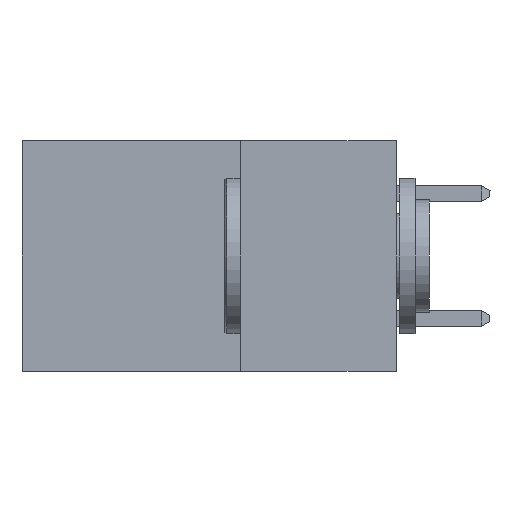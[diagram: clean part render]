
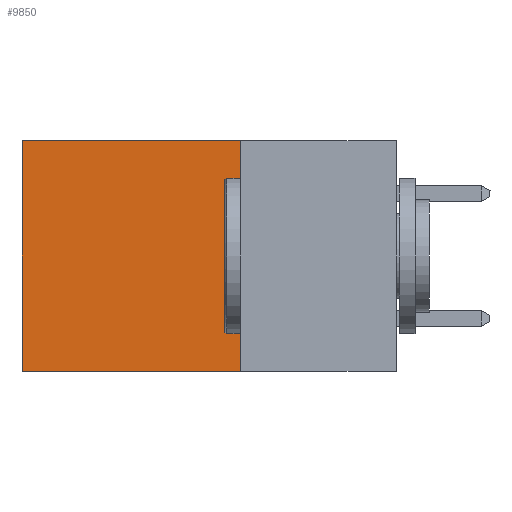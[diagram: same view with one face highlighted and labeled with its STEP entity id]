
A CAD part, left-side view. The second image highlights one B-rep face of the part: STEP entity #9850.
In plain terms, the highlighted planar face has unit normal (-1, 0, 0).
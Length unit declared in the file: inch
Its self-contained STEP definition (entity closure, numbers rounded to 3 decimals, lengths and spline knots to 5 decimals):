
#360 = EDGE_LOOP ( 'NONE', ( #5847, #7044, #11346, #6900 ) ) ;
#892 = DIRECTION ( 'NONE',  ( 1., 0., 0. ) ) ;
#955 = LINE ( 'NONE', #7389, #6560 ) ;
#984 = VERTEX_POINT ( 'NONE', #8014 ) ;
#1682 = AXIS2_PLACEMENT_3D ( 'NONE', #8633, #892, #7744 ) ;
#2180 = CARTESIAN_POINT ( 'NONE',  ( 0.298, 0.25, 0. ) ) ;
#2944 = EDGE_CURVE ( 'NONE', #7789, #984, #8192, .T. ) ;
#3063 = CARTESIAN_POINT ( 'NONE',  ( 0.298, 0.25, 0. ) ) ;
#3482 = LINE ( 'NONE', #5818, #8263 ) ;
#4239 = LINE ( 'NONE', #2180, #6195 ) ;
#5123 = VERTEX_POINT ( 'NONE', #5521 ) ;
#5280 = EDGE_CURVE ( 'NONE', #8466, #7789, #955, .T. ) ;
#5521 = CARTESIAN_POINT ( 'NONE',  ( 0.298, 0.25, -0.37 ) ) ;
#5671 = DIRECTION ( 'NONE',  ( 0., 0., -1. ) ) ;
#5818 = CARTESIAN_POINT ( 'NONE',  ( 0.298, 0.25, -0.37 ) ) ;
#5847 = ORIENTED_EDGE ( 'NONE', *, *, #2944, .T. ) ;
#6195 = VECTOR ( 'NONE', #7963, 39.37008 ) ;
#6253 = CARTESIAN_POINT ( 'NONE',  ( 0.298, 0.6, 0. ) ) ;
#6560 = VECTOR ( 'NONE', #9180, 39.37008 ) ;
#6900 = ORIENTED_EDGE ( 'NONE', *, *, #5280, .T. ) ;
#6981 = FACE_OUTER_BOUND ( 'NONE', #360, .T. ) ;
#7044 = ORIENTED_EDGE ( 'NONE', *, *, #10268, .F. ) ;
#7389 = CARTESIAN_POINT ( 'NONE',  ( 0.298, 0.25, 0. ) ) ;
#7744 = DIRECTION ( 'NONE',  ( 0., 0., -1. ) ) ;
#7789 = VERTEX_POINT ( 'NONE', #9794 ) ;
#7963 = DIRECTION ( 'NONE',  ( 0., 0., -1. ) ) ;
#8014 = CARTESIAN_POINT ( 'NONE',  ( 0.298, 0.6, -0.37 ) ) ;
#8192 = LINE ( 'NONE', #6253, #9104 ) ;
#8263 = VECTOR ( 'NONE', #10563, 39.37008 ) ;
#8466 = VERTEX_POINT ( 'NONE', #3063 ) ;
#8633 = CARTESIAN_POINT ( 'NONE',  ( 0.298, 0.25, 0. ) ) ;
#9104 = VECTOR ( 'NONE', #5671, 39.37008 ) ;
#9180 = DIRECTION ( 'NONE',  ( 0., 1., 0. ) ) ;
#9794 = CARTESIAN_POINT ( 'NONE',  ( 0.298, 0.6, 0. ) ) ;
#9850 = ADVANCED_FACE ( 'NONE', ( #6981 ), #12462, .F. ) ;
#10268 = EDGE_CURVE ( 'NONE', #5123, #984, #3482, .T. ) ;
#10563 = DIRECTION ( 'NONE',  ( 0., 1., 0. ) ) ;
#11346 = ORIENTED_EDGE ( 'NONE', *, *, #11757, .F. ) ;
#11757 = EDGE_CURVE ( 'NONE', #8466, #5123, #4239, .T. ) ;
#12462 = PLANE ( 'NONE',  #1682 ) ;
